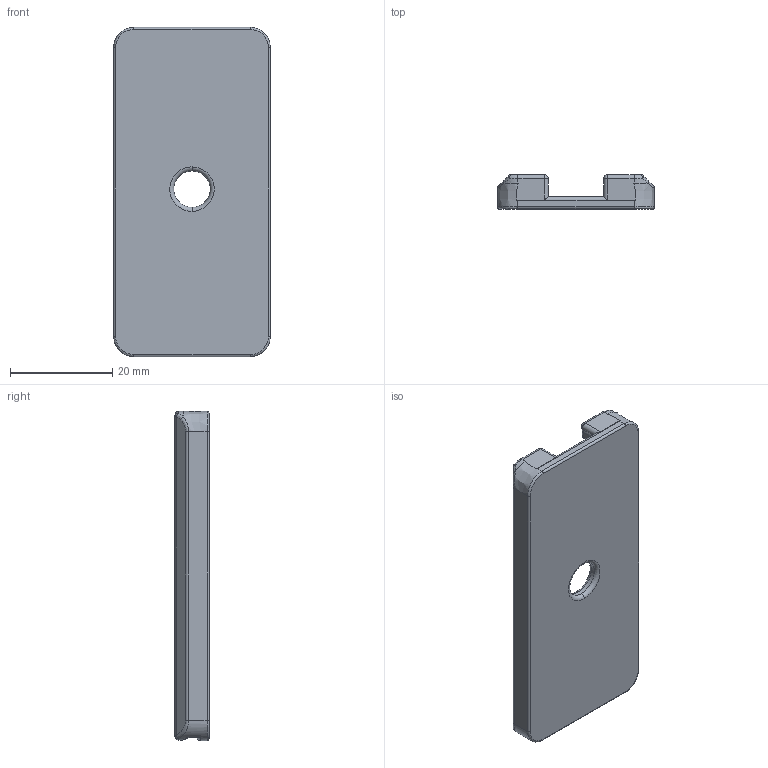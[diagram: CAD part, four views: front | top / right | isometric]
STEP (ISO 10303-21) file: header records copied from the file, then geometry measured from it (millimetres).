
FILE_DESCRIPTION(/* description */ ('STEP AP214'),/* implementation_level */ '2;1');
FILE_NAME(/* name */ 'Ivan''Ivan''s Standard Mag Baseplate.stp',/* time_stamp */ '2019-01-27T20:55:21-06:00',/* author */ ('johne'),/* organization */ (''),/* preprocessor_version */ 'ST-DEVELOPER v16.13',/* originating_system */ 'Autodesk Inventor 2018',/* authorisation */ '');
FILE_SCHEMA (('AUTOMOTIVE_DESIGN { 1 0 10303 214 3 1 1 }'));
Length unit declared in the file: millimetre
Products named in the file (1): DefDist_Cuomo_AR15_30_Mag_Base_Plate
Bounding box: 30.68 x 6.68 x 64.52 mm (x, y, z)
Volume: 6239.1 mm3; surface area: 5541.7 mm2
Topology: 1 solids, 1 shells, 101 faces, 252 edges, 151 vertices
Faces by surface type: cylinder 38, plane 25, bspline 16, torus 16, sphere 6
Full cylindrical faces by diameter (mm): 7.137 x1
Entity records: 5611 total; most frequent: CARTESIAN_POINT 3261, ORIENTED_EDGE 498, DIRECTION 481, EDGE_CURVE 249, AXIS2_PLACEMENT_3D 193, VERTEX_POINT 151, EDGE_LOOP 104, FACE_OUTER_BOUND 101
